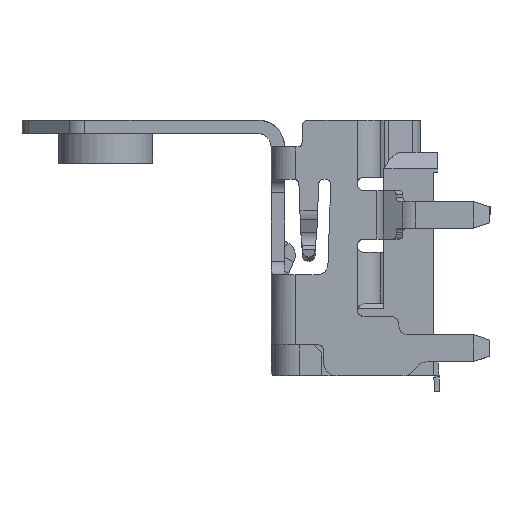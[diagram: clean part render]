
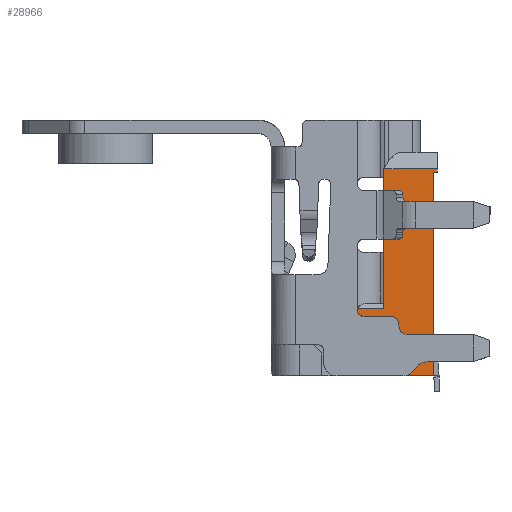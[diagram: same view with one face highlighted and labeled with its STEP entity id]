
A CAD part, left-side view. The second image highlights one B-rep face of the part: STEP entity #28966.
In plain terms, the highlighted planar face has unit normal (-1, 0, 0).
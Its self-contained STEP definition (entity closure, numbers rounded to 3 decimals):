
#2014 = ORIENTED_EDGE ( 'NONE', *, *, #54751, .T. ) ;
#2372 = EDGE_CURVE ( 'NONE', #11778, #37945, #54470, .T. ) ;
#2766 = CARTESIAN_POINT ( 'NONE',  ( -6.95, 4.994, 1.415 ) ) ;
#3289 = DIRECTION ( 'NONE',  ( 0., -1., 0. ) ) ;
#4120 = CARTESIAN_POINT ( 'NONE',  ( -6.95, -0.2, 1.415 ) ) ;
#6277 = EDGE_LOOP ( 'NONE', ( #2014, #20956, #7356, #33582, #12916, #25924, #53336, #44114 ) ) ;
#6429 = CARTESIAN_POINT ( 'NONE',  ( -6.95, -2.7, 0.84 ) ) ;
#7356 = ORIENTED_EDGE ( 'NONE', *, *, #40911, .F. ) ;
#11778 = VERTEX_POINT ( 'NONE', #11887 ) ;
#11887 = CARTESIAN_POINT ( 'NONE',  ( -6.95, 4.994, 3.405 ) ) ;
#12150 = LINE ( 'NONE', #46005, #19891 ) ;
#12914 = CARTESIAN_POINT ( 'NONE',  ( -6.95, -2.854, -1.828 ) ) ;
#12916 = ORIENTED_EDGE ( 'NONE', *, *, #57391, .T. ) ;
#13907 = VERTEX_POINT ( 'NONE', #14124 ) ;
#14124 = CARTESIAN_POINT ( 'NONE',  ( -6.95, 4.85, 3.405 ) ) ;
#17315 = VERTEX_POINT ( 'NONE', #49753 ) ;
#18212 = DIRECTION ( 'NONE',  ( 0., 0., -1. ) ) ;
#18914 = CARTESIAN_POINT ( 'NONE',  ( -6.95, 1.147, -0.195 ) ) ;
#19891 = VECTOR ( 'NONE', #21869, 1000. ) ;
#20404 = VECTOR ( 'NONE', #3289, 1000. ) ;
#20483 = VECTOR ( 'NONE', #21431, 1000. ) ;
#20956 = ORIENTED_EDGE ( 'NONE', *, *, #58607, .T. ) ;
#21431 = DIRECTION ( 'NONE',  ( 0., 1., 0. ) ) ;
#21435 = LINE ( 'NONE', #6429, #55663 ) ;
#21869 = DIRECTION ( 'NONE',  ( 0., -1., 0. ) ) ;
#25483 = VECTOR ( 'NONE', #55622, 1000. ) ;
#25924 = ORIENTED_EDGE ( 'NONE', *, *, #2372, .T. ) ;
#26629 = EDGE_CURVE ( 'NONE', #26653, #55314, #55829, .T. ) ;
#26653 = VERTEX_POINT ( 'NONE', #4120 ) ;
#27639 = FACE_OUTER_BOUND ( 'NONE', #6277, .T. ) ;
#28239 = DIRECTION ( 'NONE',  ( -1., 0., 0. ) ) ;
#28966 = ADVANCED_FACE ( 'NONE', ( #27639 ), #61459, .T. ) ;
#30646 = VERTEX_POINT ( 'NONE', #32313 ) ;
#30888 = AXIS2_PLACEMENT_3D ( 'NONE', #12914, #28239, #46743 ) ;
#32313 = CARTESIAN_POINT ( 'NONE',  ( -6.95, 4.85, 3.255 ) ) ;
#32621 = CARTESIAN_POINT ( 'NONE',  ( -6.95, -0.2, 0.84 ) ) ;
#33582 = ORIENTED_EDGE ( 'NONE', *, *, #42994, .T. ) ;
#33668 = CARTESIAN_POINT ( 'NONE',  ( -6.95, 1.075, 3.255 ) ) ;
#33926 = EDGE_CURVE ( 'NONE', #37945, #26653, #12150, .T. ) ;
#34957 = DIRECTION ( 'NONE',  ( 0., 0., 1. ) ) ;
#35271 = LINE ( 'NONE', #40893, #25483 ) ;
#36800 = LINE ( 'NONE', #50916, #20483 ) ;
#37945 = VERTEX_POINT ( 'NONE', #2766 ) ;
#40893 = CARTESIAN_POINT ( 'NONE',  ( -6.95, 4.85, 0.84 ) ) ;
#40911 = EDGE_CURVE ( 'NONE', #30646, #17315, #57489, .T. ) ;
#42057 = VECTOR ( 'NONE', #59467, 1000. ) ;
#42994 = EDGE_CURVE ( 'NONE', #30646, #13907, #35271, .T. ) ;
#43283 = CARTESIAN_POINT ( 'NONE',  ( -6.95, -2.7, -0.195 ) ) ;
#44114 = ORIENTED_EDGE ( 'NONE', *, *, #26629, .T. ) ;
#44350 = VECTOR ( 'NONE', #52785, 1000. ) ;
#44749 = VERTEX_POINT ( 'NONE', #43283 ) ;
#46005 = CARTESIAN_POINT ( 'NONE',  ( -6.95, 1.147, 1.415 ) ) ;
#46338 = CARTESIAN_POINT ( 'NONE',  ( -6.95, -0.2, -0.195 ) ) ;
#46743 = DIRECTION ( 'NONE',  ( 0., 0., 1. ) ) ;
#49753 = CARTESIAN_POINT ( 'NONE',  ( -6.95, -2.7, 3.255 ) ) ;
#50916 = CARTESIAN_POINT ( 'NONE',  ( -6.95, 1.147, 3.405 ) ) ;
#51836 = LINE ( 'NONE', #18914, #20404 ) ;
#52785 = DIRECTION ( 'NONE',  ( 0., -1., 0. ) ) ;
#53336 = ORIENTED_EDGE ( 'NONE', *, *, #33926, .T. ) ;
#54470 = LINE ( 'NONE', #58868, #42057 ) ;
#54751 = EDGE_CURVE ( 'NONE', #55314, #44749, #51836, .T. ) ;
#55314 = VERTEX_POINT ( 'NONE', #46338 ) ;
#55622 = DIRECTION ( 'NONE',  ( 0., 0., 1. ) ) ;
#55663 = VECTOR ( 'NONE', #34957, 1000. ) ;
#55829 = LINE ( 'NONE', #32621, #58764 ) ;
#57391 = EDGE_CURVE ( 'NONE', #13907, #11778, #36800, .T. ) ;
#57489 = LINE ( 'NONE', #33668, #44350 ) ;
#58607 = EDGE_CURVE ( 'NONE', #44749, #17315, #21435, .T. ) ;
#58764 = VECTOR ( 'NONE', #18212, 1000. ) ;
#58868 = CARTESIAN_POINT ( 'NONE',  ( -6.95, 4.994, 0.84 ) ) ;
#59467 = DIRECTION ( 'NONE',  ( 0., 0., -1. ) ) ;
#61459 = PLANE ( 'NONE',  #30888 ) ;
